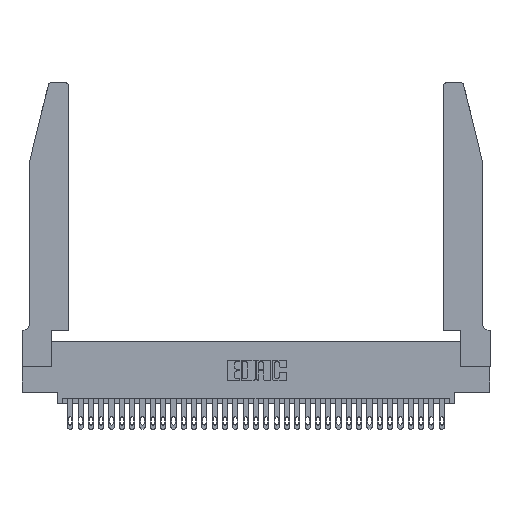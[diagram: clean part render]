
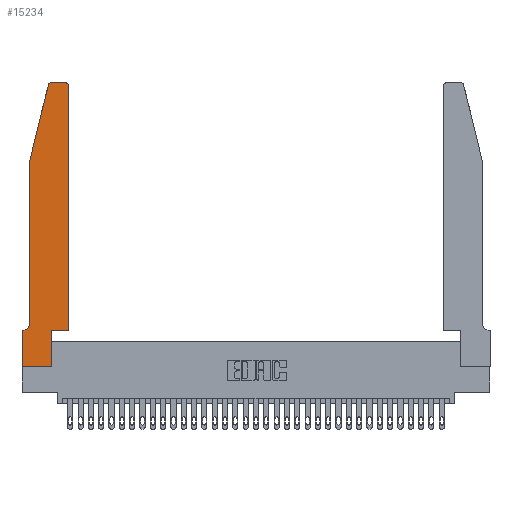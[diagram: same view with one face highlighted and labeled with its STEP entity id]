
A CAD part, top view. The second image highlights one B-rep face of the part: STEP entity #15234.
In plain terms, the highlighted planar face has unit normal (0, 0, 1).
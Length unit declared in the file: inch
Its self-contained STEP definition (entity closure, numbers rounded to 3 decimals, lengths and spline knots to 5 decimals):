
#232 = DIRECTION ( 'NONE',  ( -0.239, -0.971, 0. ) ) ;
#286 = EDGE_CURVE ( 'NONE', #9001, #12033, #5997, .T. ) ;
#529 = CARTESIAN_POINT ( 'NONE',  ( 0.4505, 0.35, 0.37 ) ) ;
#700 = CARTESIAN_POINT ( 'NONE',  ( 0.2605, 2.75, 0.37 ) ) ;
#834 = LINE ( 'NONE', #25245, #23479 ) ;
#1581 = EDGE_CURVE ( 'NONE', #12033, #21286, #10577, .T. ) ;
#2088 = CIRCLE ( 'NONE', #18669, 0.07 ) ;
#2469 = ORIENTED_EDGE ( 'NONE', *, *, #1581, .T. ) ;
#3396 = DIRECTION ( 'NONE',  ( -1., 0., 0. ) ) ;
#3419 = VECTOR ( 'NONE', #232, 39.37008 ) ;
#3524 = LINE ( 'NONE', #9872, #6034 ) ;
#3758 = CARTESIAN_POINT ( 'NONE',  ( 0.0755, 0.35, 0.37 ) ) ;
#3819 = VERTEX_POINT ( 'NONE', #4311 ) ;
#4035 = ORIENTED_EDGE ( 'NONE', *, *, #27486, .T. ) ;
#4311 = CARTESIAN_POINT ( 'NONE',  ( 0.2865, 0.35, 0.37 ) ) ;
#4654 = EDGE_CURVE ( 'NONE', #28526, #9001, #14989, .T. ) ;
#4825 = DIRECTION ( 'NONE',  ( 0., 0., -1. ) ) ;
#5376 = LINE ( 'NONE', #22058, #27537 ) ;
#5729 = CARTESIAN_POINT ( 'NONE',  ( 0.284, 2.72, 0.37 ) ) ;
#5997 = CIRCLE ( 'NONE', #16415, 0.03 ) ;
#6034 = VECTOR ( 'NONE', #21057, 39.37008 ) ;
#6076 = FACE_OUTER_BOUND ( 'NONE', #26563, .T. ) ;
#6178 = VECTOR ( 'NONE', #19406, 39.37008 ) ;
#6239 = CARTESIAN_POINT ( 'NONE',  ( 0.0055, 0.35, 0.37 ) ) ;
#6697 = EDGE_CURVE ( 'NONE', #23411, #18098, #3524, .T. ) ;
#7568 = VECTOR ( 'NONE', #3396, 39.37008 ) ;
#7932 = DIRECTION ( 'NONE',  ( 1., 0., 0. ) ) ;
#8857 = DIRECTION ( 'NONE',  ( 0., -1., 0. ) ) ;
#9001 = VERTEX_POINT ( 'NONE', #20452 ) ;
#9592 = ORIENTED_EDGE ( 'NONE', *, *, #22217, .T. ) ;
#9872 = CARTESIAN_POINT ( 'NONE',  ( 0., 0., 0.37 ) ) ;
#10092 = LINE ( 'NONE', #3758, #7568 ) ;
#10426 = LINE ( 'NONE', #18278, #22955 ) ;
#10577 = LINE ( 'NONE', #32436, #3419 ) ;
#10672 = CARTESIAN_POINT ( 'NONE',  ( 0., 0.35, 0.37 ) ) ;
#11664 = ORIENTED_EDGE ( 'NONE', *, *, #27595, .T. ) ;
#11762 = ORIENTED_EDGE ( 'NONE', *, *, #13843, .T. ) ;
#11931 = DIRECTION ( 'NONE',  ( 0., 1., 0. ) ) ;
#12033 = VERTEX_POINT ( 'NONE', #24815 ) ;
#12101 = ORIENTED_EDGE ( 'NONE', *, *, #286, .T. ) ;
#12924 = ORIENTED_EDGE ( 'NONE', *, *, #19563, .T. ) ;
#13332 = DIRECTION ( 'NONE',  ( 0., 0., 1. ) ) ;
#13422 = CARTESIAN_POINT ( 'NONE',  ( 0.4205, 2.72, 0.37 ) ) ;
#13843 = EDGE_CURVE ( 'NONE', #3819, #24711, #22440, .T. ) ;
#14989 = LINE ( 'NONE', #700, #6178 ) ;
#15020 = VERTEX_POINT ( 'NONE', #6239 ) ;
#15234 = ADVANCED_FACE ( 'NONE', ( #6076 ), #23165, .T. ) ;
#15389 = CARTESIAN_POINT ( 'NONE',  ( 0.2865, 0., 0.37 ) ) ;
#16415 = AXIS2_PLACEMENT_3D ( 'NONE', #5729, #29560, #29459 ) ;
#17435 = AXIS2_PLACEMENT_3D ( 'NONE', #13422, #24058, #7932 ) ;
#17892 = CARTESIAN_POINT ( 'NONE',  ( 0.4205, 2.75, 0.37 ) ) ;
#18098 = VERTEX_POINT ( 'NONE', #15389 ) ;
#18278 = CARTESIAN_POINT ( 'NONE',  ( 0.0755, 2., 0.37 ) ) ;
#18669 = AXIS2_PLACEMENT_3D ( 'NONE', #31457, #4825, #25841 ) ;
#19069 = VECTOR ( 'NONE', #27461, 39.37008 ) ;
#19073 = CARTESIAN_POINT ( 'NONE',  ( 0., 0., 0.37 ) ) ;
#19133 = EDGE_CURVE ( 'NONE', #24998, #23411, #5376, .T. ) ;
#19160 = CARTESIAN_POINT ( 'NONE',  ( 0.0755, 0.42, 0.37 ) ) ;
#19163 = DIRECTION ( 'NONE',  ( 0., -1., 0. ) ) ;
#19406 = DIRECTION ( 'NONE',  ( -1., 0., 0. ) ) ;
#19563 = EDGE_CURVE ( 'NONE', #21286, #33184, #10426, .T. ) ;
#20452 = CARTESIAN_POINT ( 'NONE',  ( 0.284, 2.75, 0.37 ) ) ;
#21057 = DIRECTION ( 'NONE',  ( 1., 0., 0. ) ) ;
#21286 = VERTEX_POINT ( 'NONE', #25767 ) ;
#21313 = AXIS2_PLACEMENT_3D ( 'NONE', #30341, #13332, #22870 ) ;
#21922 = VERTEX_POINT ( 'NONE', #23880 ) ;
#22058 = CARTESIAN_POINT ( 'NONE',  ( 0., 0., 0.37 ) ) ;
#22062 = ORIENTED_EDGE ( 'NONE', *, *, #30920, .T. ) ;
#22217 = EDGE_CURVE ( 'NONE', #24711, #21922, #834, .T. ) ;
#22382 = CIRCLE ( 'NONE', #17435, 0.03 ) ;
#22440 = LINE ( 'NONE', #30381, #19069 ) ;
#22870 = DIRECTION ( 'NONE',  ( 1., 0., 0. ) ) ;
#22955 = VECTOR ( 'NONE', #19163, 39.37008 ) ;
#23165 = PLANE ( 'NONE',  #21313 ) ;
#23411 = VERTEX_POINT ( 'NONE', #19073 ) ;
#23479 = VECTOR ( 'NONE', #11931, 39.37008 ) ;
#23502 = DIRECTION ( 'NONE',  ( 0., 1., 0. ) ) ;
#23880 = CARTESIAN_POINT ( 'NONE',  ( 0.4505, 2.72, 0.37 ) ) ;
#24058 = DIRECTION ( 'NONE',  ( 0., 0., 1. ) ) ;
#24089 = ORIENTED_EDGE ( 'NONE', *, *, #4654, .T. ) ;
#24711 = VERTEX_POINT ( 'NONE', #529 ) ;
#24815 = CARTESIAN_POINT ( 'NONE',  ( 0.25487, 2.72718, 0.37 ) ) ;
#24998 = VERTEX_POINT ( 'NONE', #10672 ) ;
#25245 = CARTESIAN_POINT ( 'NONE',  ( 0.4505, 0.35, 0.37 ) ) ;
#25767 = CARTESIAN_POINT ( 'NONE',  ( 0.0755, 2., 0.37 ) ) ;
#25841 = DIRECTION ( 'NONE',  ( -1., 0., 0. ) ) ;
#25934 = CARTESIAN_POINT ( 'NONE',  ( 0.2865, 0.35, 0.37 ) ) ;
#26563 = EDGE_LOOP ( 'NONE', ( #24089, #12101, #2469, #12924, #22062, #34420, #32757, #29454, #4035, #11762, #9592, #11664 ) ) ;
#27461 = DIRECTION ( 'NONE',  ( 1., 0., 0. ) ) ;
#27486 = EDGE_CURVE ( 'NONE', #18098, #3819, #31596, .T. ) ;
#27537 = VECTOR ( 'NONE', #8857, 39.37008 ) ;
#27595 = EDGE_CURVE ( 'NONE', #21922, #28526, #22382, .T. ) ;
#28526 = VERTEX_POINT ( 'NONE', #17892 ) ;
#29454 = ORIENTED_EDGE ( 'NONE', *, *, #6697, .T. ) ;
#29459 = DIRECTION ( 'NONE',  ( 1., 0., 0. ) ) ;
#29560 = DIRECTION ( 'NONE',  ( 0., 0., 1. ) ) ;
#30341 = CARTESIAN_POINT ( 'NONE',  ( 0., 0.35, 0.37 ) ) ;
#30381 = CARTESIAN_POINT ( 'NONE',  ( 0.4505, 0.35, 0.37 ) ) ;
#30743 = VECTOR ( 'NONE', #23502, 39.37008 ) ;
#30920 = EDGE_CURVE ( 'NONE', #33184, #15020, #2088, .T. ) ;
#31457 = CARTESIAN_POINT ( 'NONE',  ( 0.0055, 0.42, 0.37 ) ) ;
#31596 = LINE ( 'NONE', #25934, #30743 ) ;
#32436 = CARTESIAN_POINT ( 'NONE',  ( 0.0755, 2., 0.37 ) ) ;
#32757 = ORIENTED_EDGE ( 'NONE', *, *, #19133, .T. ) ;
#33184 = VERTEX_POINT ( 'NONE', #19160 ) ;
#34369 = EDGE_CURVE ( 'NONE', #15020, #24998, #10092, .T. ) ;
#34420 = ORIENTED_EDGE ( 'NONE', *, *, #34369, .T. ) ;
